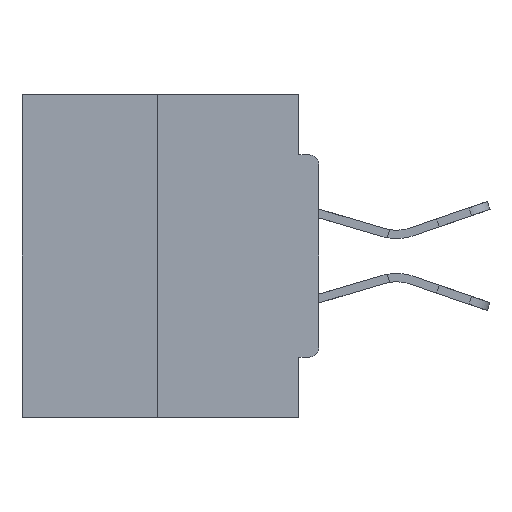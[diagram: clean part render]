
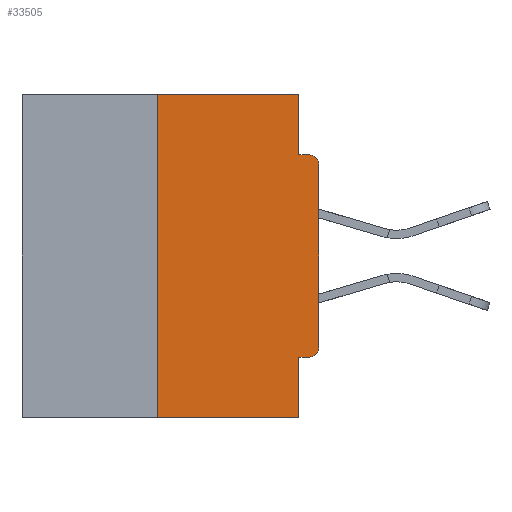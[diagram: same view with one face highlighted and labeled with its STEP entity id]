
A CAD part, left-side view. The second image highlights one B-rep face of the part: STEP entity #33505.
In plain terms, the highlighted planar face has unit normal (-1, 0, 0).
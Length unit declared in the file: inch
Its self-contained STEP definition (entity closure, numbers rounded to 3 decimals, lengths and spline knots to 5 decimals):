
#15 = ORIENTED_EDGE ( 'NONE', *, *, #3559, .T. ) ;
#136 = CARTESIAN_POINT ( 'NONE',  ( 0., 0.015, -0.3915 ) ) ;
#402 = EDGE_CURVE ( 'NONE', #15504, #15661, #4581, .T. ) ;
#565 = CARTESIAN_POINT ( 'NONE',  ( 0., 0.031, -0.5 ) ) ;
#598 = ORIENTED_EDGE ( 'NONE', *, *, #25042, .F. ) ;
#606 = EDGE_CURVE ( 'NONE', #22201, #1834, #4945, .T. ) ;
#951 = CARTESIAN_POINT ( 'NONE',  ( 0., 0.031, -0.5 ) ) ;
#1167 = ORIENTED_EDGE ( 'NONE', *, *, #606, .T. ) ;
#1298 = CARTESIAN_POINT ( 'NONE',  ( 0., 0., -0.4065 ) ) ;
#1434 = LINE ( 'NONE', #1298, #13171 ) ;
#1784 = CIRCLE ( 'NONE', #3313, 0.015 ) ;
#1834 = VERTEX_POINT ( 'NONE', #12952 ) ;
#2282 = EDGE_CURVE ( 'NONE', #19873, #22201, #8023, .T. ) ;
#2475 = CARTESIAN_POINT ( 'NONE',  ( 0., 0.031, -0.0935 ) ) ;
#3313 = AXIS2_PLACEMENT_3D ( 'NONE', #6046, #18581, #21394 ) ;
#3559 = EDGE_CURVE ( 'NONE', #1834, #28670, #1784, .T. ) ;
#3765 = VECTOR ( 'NONE', #17750, 39.37008 ) ;
#3894 = CARTESIAN_POINT ( 'NONE',  ( 0., 0.46, 0. ) ) ;
#4412 = VERTEX_POINT ( 'NONE', #951 ) ;
#4581 = LINE ( 'NONE', #11668, #5809 ) ;
#4945 = LINE ( 'NONE', #15358, #3765 ) ;
#5484 = DIRECTION ( 'NONE',  ( 0., 0., 1. ) ) ;
#5809 = VECTOR ( 'NONE', #32815, 39.37008 ) ;
#6046 = CARTESIAN_POINT ( 'NONE',  ( 0., 0.015, -0.1085 ) ) ;
#6053 = VECTOR ( 'NONE', #5484, 39.37008 ) ;
#6275 = EDGE_CURVE ( 'NONE', #25964, #4412, #10512, .T. ) ;
#8023 = CIRCLE ( 'NONE', #27990, 0.015 ) ;
#8271 = CARTESIAN_POINT ( 'NONE',  ( 0., 0.46, -0.5 ) ) ;
#8355 = ORIENTED_EDGE ( 'NONE', *, *, #2282, .T. ) ;
#8814 = ORIENTED_EDGE ( 'NONE', *, *, #402, .F. ) ;
#10512 = LINE ( 'NONE', #565, #30361 ) ;
#11182 = CARTESIAN_POINT ( 'NONE',  ( 0., 0.031, -0.4065 ) ) ;
#11668 = CARTESIAN_POINT ( 'NONE',  ( 0., 0.031, 0. ) ) ;
#12104 = LINE ( 'NONE', #20957, #6053 ) ;
#12769 = LINE ( 'NONE', #23000, #28556 ) ;
#12868 = EDGE_CURVE ( 'NONE', #15661, #28670, #12769, .T. ) ;
#12952 = CARTESIAN_POINT ( 'NONE',  ( 0., 0., -0.1085 ) ) ;
#13171 = VECTOR ( 'NONE', #26703, 39.37008 ) ;
#13526 = VECTOR ( 'NONE', #25965, 39.37008 ) ;
#13705 = VERTEX_POINT ( 'NONE', #25973 ) ;
#14303 = EDGE_LOOP ( 'NONE', ( #32080, #22698, #24148, #23275, #598, #8355, #1167, #15, #23774, #8814 ) ) ;
#15114 = FACE_OUTER_BOUND ( 'NONE', #14303, .T. ) ;
#15358 = CARTESIAN_POINT ( 'NONE',  ( 0., 0., 0. ) ) ;
#15417 = DIRECTION ( 'NONE',  ( 0., 0., -1. ) ) ;
#15504 = VERTEX_POINT ( 'NONE', #20017 ) ;
#15661 = VERTEX_POINT ( 'NONE', #2475 ) ;
#17750 = DIRECTION ( 'NONE',  ( 0., 0., 1. ) ) ;
#18216 = CARTESIAN_POINT ( 'NONE',  ( 0., 0.015, -0.0935 ) ) ;
#18581 = DIRECTION ( 'NONE',  ( -1., 0., 0. ) ) ;
#19535 = AXIS2_PLACEMENT_3D ( 'NONE', #3894, #22175, #27208 ) ;
#19873 = VERTEX_POINT ( 'NONE', #22663 ) ;
#20017 = CARTESIAN_POINT ( 'NONE',  ( 0., 0.031, 0. ) ) ;
#20398 = LINE ( 'NONE', #28356, #13526 ) ;
#20957 = CARTESIAN_POINT ( 'NONE',  ( 0., 0.25, 0. ) ) ;
#21394 = DIRECTION ( 'NONE',  ( 0., 0., -1. ) ) ;
#22175 = DIRECTION ( 'NONE',  ( 1., 0., 0. ) ) ;
#22201 = VERTEX_POINT ( 'NONE', #23723 ) ;
#22382 = PLANE ( 'NONE',  #19535 ) ;
#22512 = LINE ( 'NONE', #8271, #29869 ) ;
#22663 = CARTESIAN_POINT ( 'NONE',  ( 0., 0.015, -0.4065 ) ) ;
#22698 = ORIENTED_EDGE ( 'NONE', *, *, #23257, .F. ) ;
#23000 = CARTESIAN_POINT ( 'NONE',  ( 0., 0., -0.0935 ) ) ;
#23257 = EDGE_CURVE ( 'NONE', #13705, #27989, #12104, .T. ) ;
#23275 = ORIENTED_EDGE ( 'NONE', *, *, #6275, .F. ) ;
#23723 = CARTESIAN_POINT ( 'NONE',  ( 0., 0., -0.3915 ) ) ;
#23774 = ORIENTED_EDGE ( 'NONE', *, *, #12868, .F. ) ;
#23790 = CARTESIAN_POINT ( 'NONE',  ( 0., 0.25, 0. ) ) ;
#23956 = DIRECTION ( 'NONE',  ( 0., 0., -1. ) ) ;
#24148 = ORIENTED_EDGE ( 'NONE', *, *, #24406, .T. ) ;
#24406 = EDGE_CURVE ( 'NONE', #13705, #4412, #22512, .T. ) ;
#25042 = EDGE_CURVE ( 'NONE', #19873, #25964, #1434, .T. ) ;
#25964 = VERTEX_POINT ( 'NONE', #11182 ) ;
#25965 = DIRECTION ( 'NONE',  ( 0., -1., 0. ) ) ;
#25973 = CARTESIAN_POINT ( 'NONE',  ( 0., 0.25, -0.5 ) ) ;
#26703 = DIRECTION ( 'NONE',  ( 0., 1., 0. ) ) ;
#27203 = EDGE_CURVE ( 'NONE', #27989, #15504, #20398, .T. ) ;
#27208 = DIRECTION ( 'NONE',  ( 0., 0., -1. ) ) ;
#27989 = VERTEX_POINT ( 'NONE', #23790 ) ;
#27990 = AXIS2_PLACEMENT_3D ( 'NONE', #136, #28800, #15417 ) ;
#28356 = CARTESIAN_POINT ( 'NONE',  ( 0., 0.46, 0. ) ) ;
#28556 = VECTOR ( 'NONE', #30525, 39.37008 ) ;
#28670 = VERTEX_POINT ( 'NONE', #18216 ) ;
#28800 = DIRECTION ( 'NONE',  ( -1., 0., 0. ) ) ;
#29869 = VECTOR ( 'NONE', #32286, 39.37008 ) ;
#30361 = VECTOR ( 'NONE', #23956, 39.37008 ) ;
#30525 = DIRECTION ( 'NONE',  ( 0., -1., 0. ) ) ;
#32080 = ORIENTED_EDGE ( 'NONE', *, *, #27203, .F. ) ;
#32286 = DIRECTION ( 'NONE',  ( 0., -1., 0. ) ) ;
#32815 = DIRECTION ( 'NONE',  ( 0., 0., -1. ) ) ;
#33505 = ADVANCED_FACE ( 'NONE', ( #15114 ), #22382, .F. ) ;
